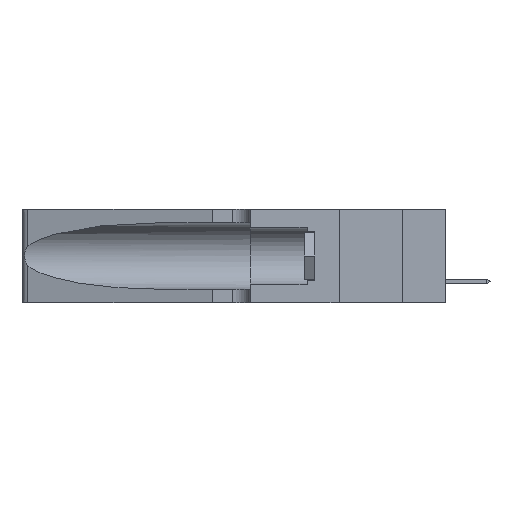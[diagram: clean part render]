
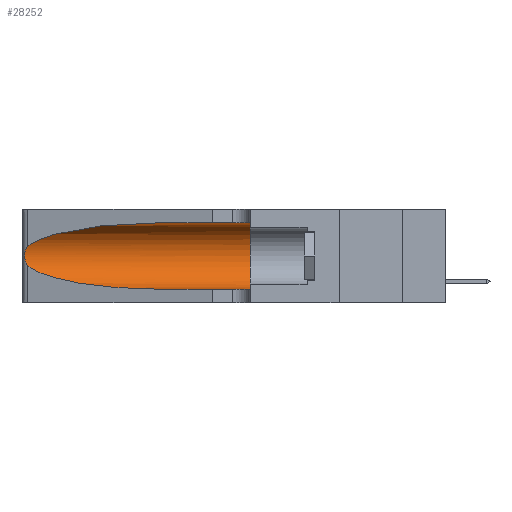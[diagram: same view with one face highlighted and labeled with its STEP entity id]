
A CAD part, left-side view. The second image highlights one B-rep face of the part: STEP entity #28252.
In plain terms, the highlighted cylindrical face has radius 3.308 mm (diameter 6.617 mm), a partial arc.
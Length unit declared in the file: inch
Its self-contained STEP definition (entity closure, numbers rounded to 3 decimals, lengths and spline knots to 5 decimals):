
#672 = CARTESIAN_POINT ( 'NONE',  ( 0.2373, 1.15595, 0.28018 ) ) ;
#1832 = CARTESIAN_POINT ( 'NONE',  ( 0.1305, 0.72297, 0.31525 ) ) ;
#3165 = CARTESIAN_POINT ( 'NONE',  ( 0.25487, 1.22718, 0.22369 ) ) ;
#3387 = CARTESIAN_POINT ( 'NONE',  ( 0.1305, 0.72297, 0.31525 ) ) ;
#3529 = CARTESIAN_POINT ( 'NONE',  ( 0.1305, 0.72297, 0.05475 ) ) ;
#3861 =( BOUNDED_CURVE ( )  B_SPLINE_CURVE ( 3, ( #3387, #15566, #672, #3165 ),
 .UNSPECIFIED., .F., .F. ) 
 B_SPLINE_CURVE_WITH_KNOTS ( ( 4, 4 ),
 ( 1.5708, 2.84003 ),
 .UNSPECIFIED. ) 
 CURVE ( )  GEOMETRIC_REPRESENTATION_ITEM ( )  RATIONAL_B_SPLINE_CURVE ( ( 1., 0.87, 0.87, 1. ) ) 
 REPRESENTATION_ITEM ( '' )  );
#4336 = B_SPLINE_CURVE_WITH_KNOTS ( 'NONE', 3,
 ( #22976, #5642, #8165, #10464, #5879, #23202, #15435, #8392, #10686, #13326, #10919, #5764, #15534, #20849 ),
 .UNSPECIFIED., .F., .F.,
 ( 4, 2, 2, 2, 2, 2, 4 ),
 ( 0., 0.00027, 0.00053, 0.00107, 0.0016, 0.00187, 0.00214 ),
 .UNSPECIFIED. ) ;
#4722 = CARTESIAN_POINT ( 'NONE',  ( 0.1305, 0.35, 0.31525 ) ) ;
#5642 = CARTESIAN_POINT ( 'NONE',  ( 0.25555, 1.22994, 0.2215 ) ) ;
#5764 = CARTESIAN_POINT ( 'NONE',  ( 0.25639, 1.23186, 0.15144 ) ) ;
#5879 = CARTESIAN_POINT ( 'NONE',  ( 0.25854, 1.2359, 0.20912 ) ) ;
#6494 = FACE_OUTER_BOUND ( 'NONE', #16164, .T. ) ;
#6518 = CARTESIAN_POINT ( 'NONE',  ( 0.1305, 1.61858, 0.31525 ) ) ;
#6700 = VERTEX_POINT ( 'NONE', #4722 ) ;
#6814 = ORIENTED_EDGE ( 'NONE', *, *, #20319, .T. ) ;
#7218 = EDGE_CURVE ( 'NONE', #6700, #22487, #13360, .T. ) ;
#7728 = AXIS2_PLACEMENT_3D ( 'NONE', #14856, #14528, #9646 ) ;
#8165 = CARTESIAN_POINT ( 'NONE',  ( 0.25639, 1.23184, 0.21858 ) ) ;
#8392 = CARTESIAN_POINT ( 'NONE',  ( 0.26075, 1.23896, 0.178 ) ) ;
#8415 = CARTESIAN_POINT ( 'NONE',  ( 0.25487, 1.22718, 0.22369 ) ) ;
#8992 = ORIENTED_EDGE ( 'NONE', *, *, #7218, .F. ) ;
#9646 = DIRECTION ( 'NONE',  ( 0., 0., -1. ) ) ;
#10464 = CARTESIAN_POINT ( 'NONE',  ( 0.25787, 1.23484, 0.2124 ) ) ;
#10686 = CARTESIAN_POINT ( 'NONE',  ( 0.26017, 1.23833, 0.17102 ) ) ;
#10919 = CARTESIAN_POINT ( 'NONE',  ( 0.25789, 1.23486, 0.15765 ) ) ;
#11433 = VECTOR ( 'NONE', #21292, 39.37008 ) ;
#11782 = ORIENTED_EDGE ( 'NONE', *, *, #12994, .T. ) ;
#12994 = EDGE_CURVE ( 'NONE', #26997, #14464, #4336, .T. ) ;
#13326 = CARTESIAN_POINT ( 'NONE',  ( 0.25856, 1.23593, 0.16098 ) ) ;
#13360 = CIRCLE ( 'NONE', #14536, 0.13025 ) ;
#13664 = VERTEX_POINT ( 'NONE', #1832 ) ;
#14319 = CARTESIAN_POINT ( 'NONE',  ( 0.25487, 1.22718, 0.14631 ) ) ;
#14464 = VERTEX_POINT ( 'NONE', #14319 ) ;
#14528 = DIRECTION ( 'NONE',  ( 0., -1., 0. ) ) ;
#14536 = AXIS2_PLACEMENT_3D ( 'NONE', #31022, #16195, #18806 ) ;
#14856 = CARTESIAN_POINT ( 'NONE',  ( 0.1305, 1.61858, 0.185 ) ) ;
#15435 = CARTESIAN_POINT ( 'NONE',  ( 0.26075, 1.23896, 0.19203 ) ) ;
#15534 = CARTESIAN_POINT ( 'NONE',  ( 0.25555, 1.22993, 0.14849 ) ) ;
#15566 = CARTESIAN_POINT ( 'NONE',  ( 0.18966, 0.96281, 0.31525 ) ) ;
#15635 = CARTESIAN_POINT ( 'NONE',  ( 0.1305, 0.72297, 0.05475 ) ) ;
#15931 = CARTESIAN_POINT ( 'NONE',  ( 0.25487, 1.22718, 0.14631 ) ) ;
#16164 = EDGE_LOOP ( 'NONE', ( #19223, #11782, #6814, #24177, #8992, #31584 ) ) ;
#16195 = DIRECTION ( 'NONE',  ( 0., 1., 0. ) ) ;
#18596 = CARTESIAN_POINT ( 'NONE',  ( 0.1305, 1.61858, 0.05475 ) ) ;
#18806 = DIRECTION ( 'NONE',  ( 0., 0., 1. ) ) ;
#19223 = ORIENTED_EDGE ( 'NONE', *, *, #24639, .T. ) ;
#20319 = EDGE_CURVE ( 'NONE', #14464, #20720, #22218, .T. ) ;
#20659 = LINE ( 'NONE', #18596, #11433 ) ;
#20720 = VERTEX_POINT ( 'NONE', #15635 ) ;
#20849 = CARTESIAN_POINT ( 'NONE',  ( 0.25487, 1.22718, 0.14631 ) ) ;
#21292 = DIRECTION ( 'NONE',  ( 0., -1., 0. ) ) ;
#22218 =( BOUNDED_CURVE ( )  B_SPLINE_CURVE ( 3, ( #15931, #23263, #23383, #3529 ),
 .UNSPECIFIED., .F., .F. ) 
 B_SPLINE_CURVE_WITH_KNOTS ( ( 4, 4 ),
 ( 3.44316, 4.71239 ),
 .UNSPECIFIED. ) 
 CURVE ( )  GEOMETRIC_REPRESENTATION_ITEM ( )  RATIONAL_B_SPLINE_CURVE ( ( 1., 0.87, 0.87, 1. ) ) 
 REPRESENTATION_ITEM ( '' )  );
#22233 = EDGE_CURVE ( 'NONE', #20720, #22487, #20659, .T. ) ;
#22487 = VERTEX_POINT ( 'NONE', #24931 ) ;
#22976 = CARTESIAN_POINT ( 'NONE',  ( 0.25487, 1.22718, 0.22369 ) ) ;
#23202 = CARTESIAN_POINT ( 'NONE',  ( 0.26018, 1.23835, 0.19895 ) ) ;
#23263 = CARTESIAN_POINT ( 'NONE',  ( 0.2373, 1.15595, 0.08982 ) ) ;
#23383 = CARTESIAN_POINT ( 'NONE',  ( 0.18966, 0.96281, 0.05475 ) ) ;
#23627 = EDGE_CURVE ( 'NONE', #13664, #6700, #30664, .T. ) ;
#24177 = ORIENTED_EDGE ( 'NONE', *, *, #22233, .T. ) ;
#24639 = EDGE_CURVE ( 'NONE', #13664, #26997, #3861, .T. ) ;
#24931 = CARTESIAN_POINT ( 'NONE',  ( 0.1305, 0.35, 0.05475 ) ) ;
#26997 = VERTEX_POINT ( 'NONE', #8415 ) ;
#28252 = ADVANCED_FACE ( 'NONE', ( #6494 ), #30487, .F. ) ;
#28905 = DIRECTION ( 'NONE',  ( 0., -1., 0. ) ) ;
#29883 = VECTOR ( 'NONE', #28905, 39.37008 ) ;
#30487 = CYLINDRICAL_SURFACE ( 'NONE', #7728, 0.13025 ) ;
#30664 = LINE ( 'NONE', #6518, #29883 ) ;
#31022 = CARTESIAN_POINT ( 'NONE',  ( 0.1305, 0.35, 0.185 ) ) ;
#31584 = ORIENTED_EDGE ( 'NONE', *, *, #23627, .F. ) ;
